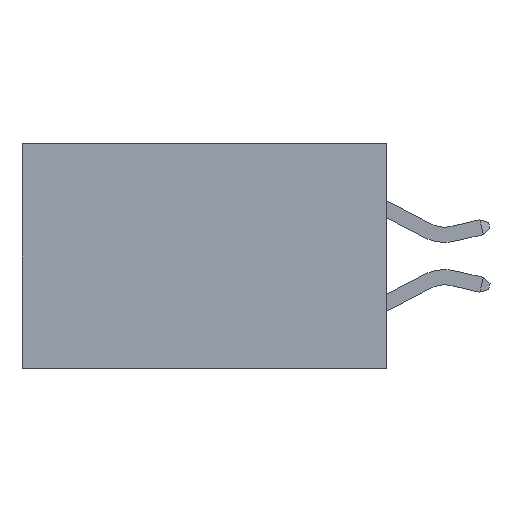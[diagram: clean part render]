
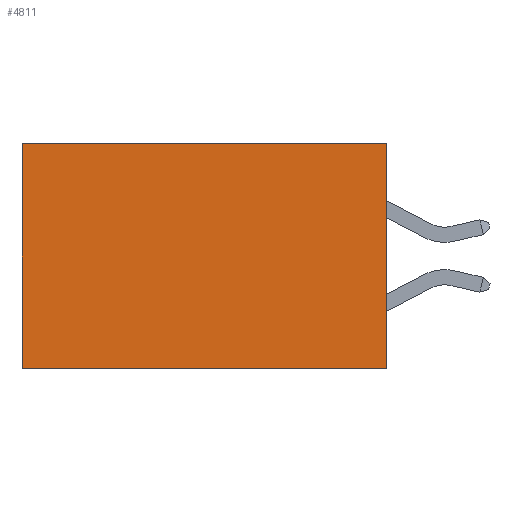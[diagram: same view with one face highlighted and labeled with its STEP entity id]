
A CAD part, left-side view. The second image highlights one B-rep face of the part: STEP entity #4811.
In plain terms, the highlighted planar face has unit normal (-1, 0, 0).
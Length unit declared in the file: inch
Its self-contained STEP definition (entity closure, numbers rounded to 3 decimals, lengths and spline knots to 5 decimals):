
#1 = LINE ( 'NONE', #12222, #9697 ) ;
#104 = ORIENTED_EDGE ( 'NONE', *, *, #6328, .F. ) ;
#442 = CARTESIAN_POINT ( 'NONE',  ( 0.2615, 0., -0.37 ) ) ;
#716 = FACE_OUTER_BOUND ( 'NONE', #6432, .T. ) ;
#900 = VECTOR ( 'NONE', #6400, 39.37008 ) ;
#2090 = EDGE_CURVE ( 'NONE', #8370, #10935, #5384, .T. ) ;
#2270 = ORIENTED_EDGE ( 'NONE', *, *, #2090, .T. ) ;
#2412 = EDGE_CURVE ( 'NONE', #10935, #11649, #8893, .T. ) ;
#3168 = CARTESIAN_POINT ( 'NONE',  ( 0.2615, 0.6, -0.37 ) ) ;
#4007 = EDGE_CURVE ( 'NONE', #8370, #7554, #5392, .T. ) ;
#4811 = ADVANCED_FACE ( 'NONE', ( #716 ), #10070, .F. ) ;
#5081 = VECTOR ( 'NONE', #7092, 39.37008 ) ;
#5170 = ORIENTED_EDGE ( 'NONE', *, *, #2412, .T. ) ;
#5384 = LINE ( 'NONE', #7065, #5081 ) ;
#5392 = LINE ( 'NONE', #7431, #7958 ) ;
#5821 = AXIS2_PLACEMENT_3D ( 'NONE', #6912, #6407, #6245 ) ;
#6245 = DIRECTION ( 'NONE',  ( 0., 0., -1. ) ) ;
#6270 = CARTESIAN_POINT ( 'NONE',  ( 0.2615, 0., 0. ) ) ;
#6328 = EDGE_CURVE ( 'NONE', #7554, #11649, #1, .T. ) ;
#6400 = DIRECTION ( 'NONE',  ( 0., 0., -1. ) ) ;
#6407 = DIRECTION ( 'NONE',  ( 1., 0., 0. ) ) ;
#6416 = CARTESIAN_POINT ( 'NONE',  ( 0.2615, 0.6, -0.37 ) ) ;
#6432 = EDGE_LOOP ( 'NONE', ( #5170, #104, #7601, #2270 ) ) ;
#6912 = CARTESIAN_POINT ( 'NONE',  ( 0.2615, 0., -0.37 ) ) ;
#7065 = CARTESIAN_POINT ( 'NONE',  ( 0.2615, 0., 0. ) ) ;
#7092 = DIRECTION ( 'NONE',  ( 0., 1., 0. ) ) ;
#7408 = DIRECTION ( 'NONE',  ( 0., 0., -1. ) ) ;
#7431 = CARTESIAN_POINT ( 'NONE',  ( 0.2615, 0., -0.37 ) ) ;
#7554 = VERTEX_POINT ( 'NONE', #442 ) ;
#7601 = ORIENTED_EDGE ( 'NONE', *, *, #4007, .F. ) ;
#7958 = VECTOR ( 'NONE', #7408, 39.37008 ) ;
#8370 = VERTEX_POINT ( 'NONE', #6270 ) ;
#8669 = CARTESIAN_POINT ( 'NONE',  ( 0.2615, 0.6, 0. ) ) ;
#8893 = LINE ( 'NONE', #6416, #900 ) ;
#9697 = VECTOR ( 'NONE', #12420, 39.37008 ) ;
#10070 = PLANE ( 'NONE',  #5821 ) ;
#10935 = VERTEX_POINT ( 'NONE', #8669 ) ;
#11649 = VERTEX_POINT ( 'NONE', #3168 ) ;
#12222 = CARTESIAN_POINT ( 'NONE',  ( 0.2615, 0., -0.37 ) ) ;
#12420 = DIRECTION ( 'NONE',  ( 0., 1., 0. ) ) ;
